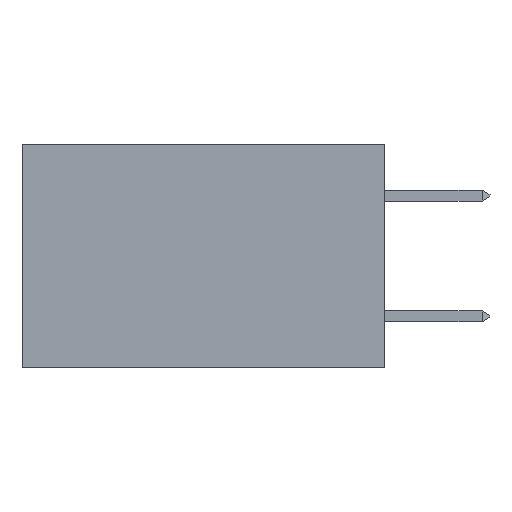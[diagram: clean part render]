
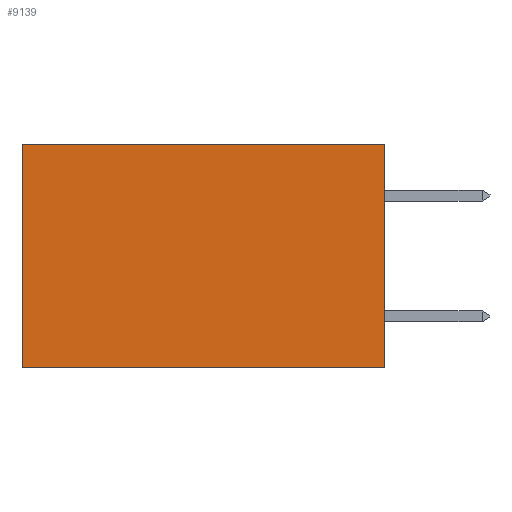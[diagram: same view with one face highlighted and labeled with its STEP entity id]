
A CAD part, left-side view. The second image highlights one B-rep face of the part: STEP entity #9139.
In plain terms, the highlighted planar face has unit normal (-1, 0, 0).
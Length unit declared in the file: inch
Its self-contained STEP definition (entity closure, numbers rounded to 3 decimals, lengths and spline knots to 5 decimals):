
#134 = EDGE_CURVE ( 'NONE', #4954, #10045, #9936, .T. ) ;
#338 = CARTESIAN_POINT ( 'NONE',  ( 0.2875, 0., 0. ) ) ;
#349 = VECTOR ( 'NONE', #6844, 39.37008 ) ;
#643 = EDGE_CURVE ( 'NONE', #10045, #21935, #9916, .T. ) ;
#896 = CARTESIAN_POINT ( 'NONE',  ( 0.2875, 0., -0.37 ) ) ;
#1572 = EDGE_CURVE ( 'NONE', #14836, #21935, #1775, .T. ) ;
#1775 = LINE ( 'NONE', #7064, #349 ) ;
#2802 = VECTOR ( 'NONE', #16908, 39.37008 ) ;
#2863 = CARTESIAN_POINT ( 'NONE',  ( 0.2875, 0., 0. ) ) ;
#3208 = CARTESIAN_POINT ( 'NONE',  ( 0.2875, 0.6, -0.37 ) ) ;
#3854 = FACE_OUTER_BOUND ( 'NONE', #20010, .T. ) ;
#3878 = DIRECTION ( 'NONE',  ( 0., 0., -1. ) ) ;
#4954 = VERTEX_POINT ( 'NONE', #2863 ) ;
#5240 = DIRECTION ( 'NONE',  ( 0., 1., 0. ) ) ;
#6664 = ORIENTED_EDGE ( 'NONE', *, *, #1572, .T. ) ;
#6844 = DIRECTION ( 'NONE',  ( 0., 0., -1. ) ) ;
#7064 = CARTESIAN_POINT ( 'NONE',  ( 0.2875, 0.6, 0. ) ) ;
#7672 = VECTOR ( 'NONE', #5240, 39.37008 ) ;
#8620 = DIRECTION ( 'NONE',  ( 1., 0., 0. ) ) ;
#9139 = ADVANCED_FACE ( 'NONE', ( #3854 ), #19246, .F. ) ;
#9179 = ORIENTED_EDGE ( 'NONE', *, *, #643, .F. ) ;
#9351 = CARTESIAN_POINT ( 'NONE',  ( 0.2875, 0., -0.37 ) ) ;
#9916 = LINE ( 'NONE', #896, #7672 ) ;
#9936 = LINE ( 'NONE', #338, #21867 ) ;
#10045 = VERTEX_POINT ( 'NONE', #9351 ) ;
#10334 = CARTESIAN_POINT ( 'NONE',  ( 0.2875, 0., 0. ) ) ;
#14201 = EDGE_CURVE ( 'NONE', #4954, #14836, #22583, .T. ) ;
#14247 = ORIENTED_EDGE ( 'NONE', *, *, #134, .F. ) ;
#14836 = VERTEX_POINT ( 'NONE', #20409 ) ;
#16908 = DIRECTION ( 'NONE',  ( 0., 1., 0. ) ) ;
#18448 = CARTESIAN_POINT ( 'NONE',  ( 0.2875, 0., 0. ) ) ;
#19246 = PLANE ( 'NONE',  #19735 ) ;
#19735 = AXIS2_PLACEMENT_3D ( 'NONE', #10334, #8620, #21037 ) ;
#20010 = EDGE_LOOP ( 'NONE', ( #6664, #9179, #14247, #21320 ) ) ;
#20409 = CARTESIAN_POINT ( 'NONE',  ( 0.2875, 0.6, 0. ) ) ;
#21037 = DIRECTION ( 'NONE',  ( 0., 0., -1. ) ) ;
#21320 = ORIENTED_EDGE ( 'NONE', *, *, #14201, .T. ) ;
#21867 = VECTOR ( 'NONE', #3878, 39.37008 ) ;
#21935 = VERTEX_POINT ( 'NONE', #3208 ) ;
#22583 = LINE ( 'NONE', #18448, #2802 ) ;
